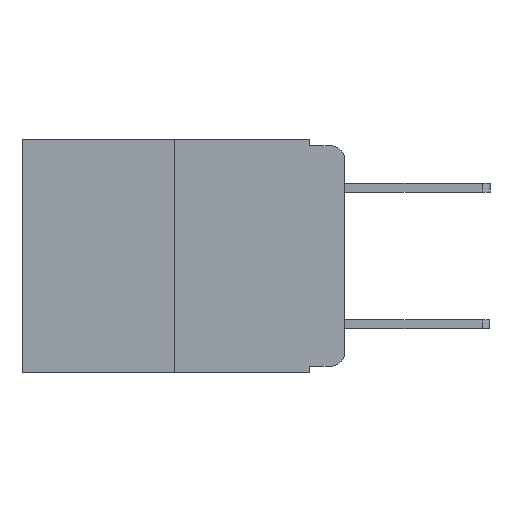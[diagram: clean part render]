
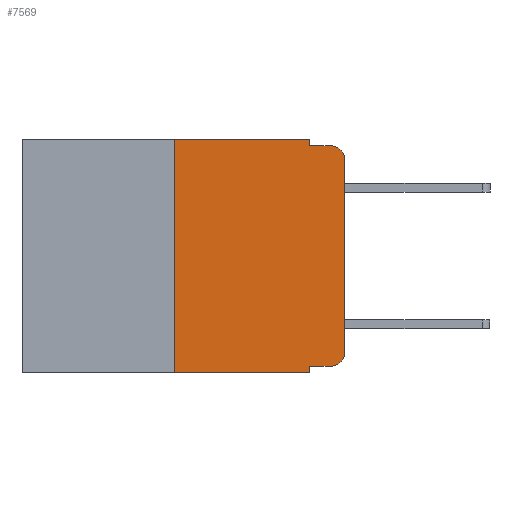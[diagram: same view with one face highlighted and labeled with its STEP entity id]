
A CAD part, left-side view. The second image highlights one B-rep face of the part: STEP entity #7569.
In plain terms, the highlighted planar face has unit normal (-1, 0, 0).
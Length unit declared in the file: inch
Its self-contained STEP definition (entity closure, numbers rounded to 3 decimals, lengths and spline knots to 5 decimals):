
#19 = CARTESIAN_POINT ( 'NONE',  ( 0., 0.02, -0.03 ) ) ;
#223 = DIRECTION ( 'NONE',  ( 0., 0., 1. ) ) ;
#238 = DIRECTION ( 'NONE',  ( -1., 0., 0. ) ) ;
#263 = LINE ( 'NONE', #2210, #10915 ) ;
#447 = VERTEX_POINT ( 'NONE', #679 ) ;
#514 = DIRECTION ( 'NONE',  ( 0., 0., -1. ) ) ;
#575 = EDGE_CURVE ( 'NONE', #5985, #839, #8918, .T. ) ;
#646 = VERTEX_POINT ( 'NONE', #2960 ) ;
#679 = CARTESIAN_POINT ( 'NONE',  ( 0., 0.02, -0.333 ) ) ;
#728 = VERTEX_POINT ( 'NONE', #10113 ) ;
#744 = CARTESIAN_POINT ( 'NONE',  ( 0., 0., -0.313 ) ) ;
#839 = VERTEX_POINT ( 'NONE', #5014 ) ;
#877 = DIRECTION ( 'NONE',  ( 0., -1., 0. ) ) ;
#904 = VECTOR ( 'NONE', #3732, 39.37008 ) ;
#912 = EDGE_LOOP ( 'NONE', ( #2415, #4838, #7361, #3026, #9549, #3307, #3905, #3353, #9387, #6059 ) ) ;
#946 = AXIS2_PLACEMENT_3D ( 'NONE', #8492, #3496, #9213 ) ;
#972 = CARTESIAN_POINT ( 'NONE',  ( 0., 0.051, -0.01 ) ) ;
#1038 = CARTESIAN_POINT ( 'NONE',  ( 0., 0.473, -0.343 ) ) ;
#1283 = EDGE_CURVE ( 'NONE', #646, #728, #7504, .T. ) ;
#1300 = CARTESIAN_POINT ( 'NONE',  ( 0., 0.051, 0. ) ) ;
#1309 = DIRECTION ( 'NONE',  ( 0., 0., -1. ) ) ;
#1543 = VERTEX_POINT ( 'NONE', #5565 ) ;
#1634 = VERTEX_POINT ( 'NONE', #9614 ) ;
#1779 = LINE ( 'NONE', #5132, #6278 ) ;
#1903 = CARTESIAN_POINT ( 'NONE',  ( 0., 0., -0.03 ) ) ;
#2210 = CARTESIAN_POINT ( 'NONE',  ( 0., 0.051, -0.333 ) ) ;
#2415 = ORIENTED_EDGE ( 'NONE', *, *, #4992, .T. ) ;
#2470 = VECTOR ( 'NONE', #1309, 39.37008 ) ;
#2562 = EDGE_CURVE ( 'NONE', #10025, #1634, #9878, .T. ) ;
#2960 = CARTESIAN_POINT ( 'NONE',  ( 0., 0.25, -0.343 ) ) ;
#3026 = ORIENTED_EDGE ( 'NONE', *, *, #2562, .F. ) ;
#3307 = ORIENTED_EDGE ( 'NONE', *, *, #1283, .F. ) ;
#3353 = ORIENTED_EDGE ( 'NONE', *, *, #575, .F. ) ;
#3383 = DIRECTION ( 'NONE',  ( 0., 0., -1. ) ) ;
#3496 = DIRECTION ( 'NONE',  ( -1., 0., 0. ) ) ;
#3643 = VERTEX_POINT ( 'NONE', #744 ) ;
#3732 = DIRECTION ( 'NONE',  ( 0., 0., -1. ) ) ;
#3749 = FACE_OUTER_BOUND ( 'NONE', #912, .T. ) ;
#3834 = EDGE_CURVE ( 'NONE', #1634, #1543, #7703, .T. ) ;
#3905 = ORIENTED_EDGE ( 'NONE', *, *, #7934, .T. ) ;
#4033 = DIRECTION ( 'NONE',  ( 0., -1., 0. ) ) ;
#4405 = EDGE_CURVE ( 'NONE', #9069, #1543, #8303, .T. ) ;
#4838 = ORIENTED_EDGE ( 'NONE', *, *, #4405, .T. ) ;
#4992 = EDGE_CURVE ( 'NONE', #3643, #9069, #1779, .T. ) ;
#5014 = CARTESIAN_POINT ( 'NONE',  ( 0., 0.051, -0.343 ) ) ;
#5132 = CARTESIAN_POINT ( 'NONE',  ( 0., 0., 0. ) ) ;
#5260 = AXIS2_PLACEMENT_3D ( 'NONE', #7644, #8399, #3383 ) ;
#5277 = VECTOR ( 'NONE', #223, 39.37008 ) ;
#5472 = VECTOR ( 'NONE', #4033, 39.37008 ) ;
#5490 = VECTOR ( 'NONE', #877, 39.37008 ) ;
#5565 = CARTESIAN_POINT ( 'NONE',  ( 0., 0.02, -0.01 ) ) ;
#5593 = CARTESIAN_POINT ( 'NONE',  ( 0., 0.051, 0. ) ) ;
#5985 = VERTEX_POINT ( 'NONE', #6775 ) ;
#6059 = ORIENTED_EDGE ( 'NONE', *, *, #10394, .T. ) ;
#6278 = VECTOR ( 'NONE', #8385, 39.37008 ) ;
#6467 = DIRECTION ( 'NONE',  ( 0., -1., 0. ) ) ;
#6775 = CARTESIAN_POINT ( 'NONE',  ( 0., 0.051, -0.333 ) ) ;
#6840 = PLANE ( 'NONE',  #5260 ) ;
#6845 = VECTOR ( 'NONE', #6467, 39.37008 ) ;
#7361 = ORIENTED_EDGE ( 'NONE', *, *, #3834, .F. ) ;
#7504 = LINE ( 'NONE', #8821, #5277 ) ;
#7569 = ADVANCED_FACE ( 'NONE', ( #3749 ), #6840, .F. ) ;
#7644 = CARTESIAN_POINT ( 'NONE',  ( 0., 0.473, 0. ) ) ;
#7682 = LINE ( 'NONE', #10347, #5472 ) ;
#7703 = LINE ( 'NONE', #972, #5490 ) ;
#7934 = EDGE_CURVE ( 'NONE', #646, #839, #10757, .T. ) ;
#8303 = CIRCLE ( 'NONE', #8616, 0.02 ) ;
#8385 = DIRECTION ( 'NONE',  ( 0., 0., 1. ) ) ;
#8399 = DIRECTION ( 'NONE',  ( 1., 0., 0. ) ) ;
#8492 = CARTESIAN_POINT ( 'NONE',  ( 0., 0.02, -0.313 ) ) ;
#8616 = AXIS2_PLACEMENT_3D ( 'NONE', #19, #238, #514 ) ;
#8821 = CARTESIAN_POINT ( 'NONE',  ( 0., 0.25, 0. ) ) ;
#8918 = LINE ( 'NONE', #1300, #2470 ) ;
#9069 = VERTEX_POINT ( 'NONE', #1903 ) ;
#9213 = DIRECTION ( 'NONE',  ( 0., 0., -1. ) ) ;
#9278 = EDGE_CURVE ( 'NONE', #728, #10025, #7682, .T. ) ;
#9387 = ORIENTED_EDGE ( 'NONE', *, *, #10845, .T. ) ;
#9495 = CARTESIAN_POINT ( 'NONE',  ( 0., 0.051, 0. ) ) ;
#9504 = CIRCLE ( 'NONE', #946, 0.02 ) ;
#9549 = ORIENTED_EDGE ( 'NONE', *, *, #9278, .F. ) ;
#9614 = CARTESIAN_POINT ( 'NONE',  ( 0., 0.051, -0.01 ) ) ;
#9878 = LINE ( 'NONE', #9495, #904 ) ;
#10025 = VERTEX_POINT ( 'NONE', #5593 ) ;
#10113 = CARTESIAN_POINT ( 'NONE',  ( 0., 0.25, 0. ) ) ;
#10347 = CARTESIAN_POINT ( 'NONE',  ( 0., 0.473, 0. ) ) ;
#10388 = DIRECTION ( 'NONE',  ( 0., -1., 0. ) ) ;
#10394 = EDGE_CURVE ( 'NONE', #447, #3643, #9504, .T. ) ;
#10757 = LINE ( 'NONE', #1038, #6845 ) ;
#10845 = EDGE_CURVE ( 'NONE', #5985, #447, #263, .T. ) ;
#10915 = VECTOR ( 'NONE', #10388, 39.37008 ) ;
